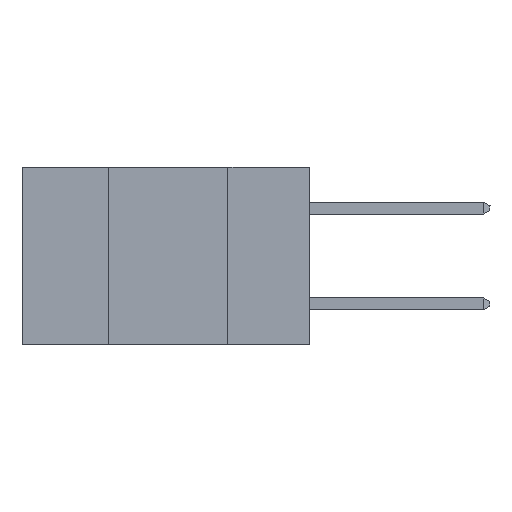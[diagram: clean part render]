
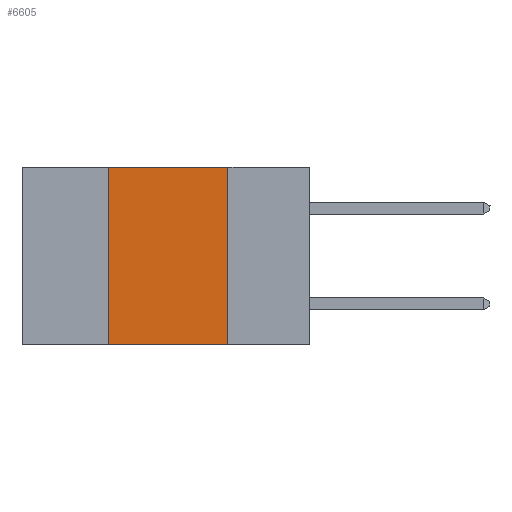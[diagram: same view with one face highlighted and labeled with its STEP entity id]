
A CAD part, left-side view. The second image highlights one B-rep face of the part: STEP entity #6605.
In plain terms, the highlighted planar face has unit normal (-1, 0, 0).
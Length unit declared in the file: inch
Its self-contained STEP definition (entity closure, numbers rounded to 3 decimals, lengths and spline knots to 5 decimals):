
#116 = VERTEX_POINT ( 'NONE', #12063 ) ;
#196 = PLANE ( 'NONE',  #14986 ) ;
#279 = EDGE_CURVE ( 'NONE', #5325, #116, #4824, .T. ) ;
#1120 = EDGE_LOOP ( 'NONE', ( #7007, #7004, #2998, #4153 ) ) ;
#1926 = FACE_OUTER_BOUND ( 'NONE', #1120, .T. ) ;
#2607 = VECTOR ( 'NONE', #18500, 39.37008 ) ;
#2998 = ORIENTED_EDGE ( 'NONE', *, *, #10888, .F. ) ;
#3368 = CARTESIAN_POINT ( 'NONE',  ( 0., 0.42, -0.37 ) ) ;
#3792 = VECTOR ( 'NONE', #7671, 39.37008 ) ;
#4153 = ORIENTED_EDGE ( 'NONE', *, *, #13429, .T. ) ;
#4824 = LINE ( 'NONE', #20639, #3792 ) ;
#5325 = VERTEX_POINT ( 'NONE', #11536 ) ;
#6605 = ADVANCED_FACE ( 'NONE', ( #1926 ), #196, .F. ) ;
#7004 = ORIENTED_EDGE ( 'NONE', *, *, #279, .F. ) ;
#7007 = ORIENTED_EDGE ( 'NONE', *, *, #19322, .F. ) ;
#7671 = DIRECTION ( 'NONE',  ( 0., -1., 0. ) ) ;
#7771 = CARTESIAN_POINT ( 'NONE',  ( 0., 0.17, -0.37 ) ) ;
#9805 = CARTESIAN_POINT ( 'NONE',  ( 0., 0.6, -0.37 ) ) ;
#10888 = EDGE_CURVE ( 'NONE', #17334, #5325, #20148, .T. ) ;
#11033 = DIRECTION ( 'NONE',  ( 1., 0., 0. ) ) ;
#11536 = CARTESIAN_POINT ( 'NONE',  ( 0., 0.42, 0. ) ) ;
#11636 = CARTESIAN_POINT ( 'NONE',  ( 0., 0.17, 0. ) ) ;
#12063 = CARTESIAN_POINT ( 'NONE',  ( 0., 0.17, 0. ) ) ;
#13429 = EDGE_CURVE ( 'NONE', #17334, #14694, #19357, .T. ) ;
#13432 = CARTESIAN_POINT ( 'NONE',  ( 0., 0.6, 0. ) ) ;
#14451 = VECTOR ( 'NONE', #14494, 39.37008 ) ;
#14494 = DIRECTION ( 'NONE',  ( 0., -1., 0. ) ) ;
#14694 = VERTEX_POINT ( 'NONE', #7771 ) ;
#14986 = AXIS2_PLACEMENT_3D ( 'NONE', #13432, #11033, #19117 ) ;
#15828 = LINE ( 'NONE', #11636, #2607 ) ;
#15934 = CARTESIAN_POINT ( 'NONE',  ( 0., 0.42, 0. ) ) ;
#17293 = VECTOR ( 'NONE', #21138, 39.37008 ) ;
#17334 = VERTEX_POINT ( 'NONE', #3368 ) ;
#18500 = DIRECTION ( 'NONE',  ( 0., 0., -1. ) ) ;
#19117 = DIRECTION ( 'NONE',  ( 0., 0., -1. ) ) ;
#19322 = EDGE_CURVE ( 'NONE', #116, #14694, #15828, .T. ) ;
#19357 = LINE ( 'NONE', #9805, #14451 ) ;
#20148 = LINE ( 'NONE', #15934, #17293 ) ;
#20639 = CARTESIAN_POINT ( 'NONE',  ( 0., 0.6, 0. ) ) ;
#21138 = DIRECTION ( 'NONE',  ( 0., 0., 1. ) ) ;
